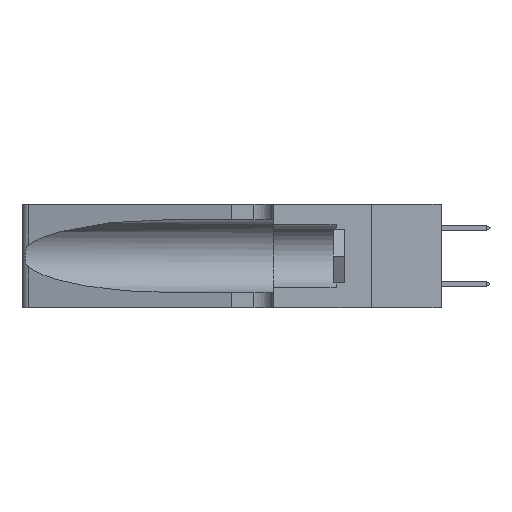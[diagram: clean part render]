
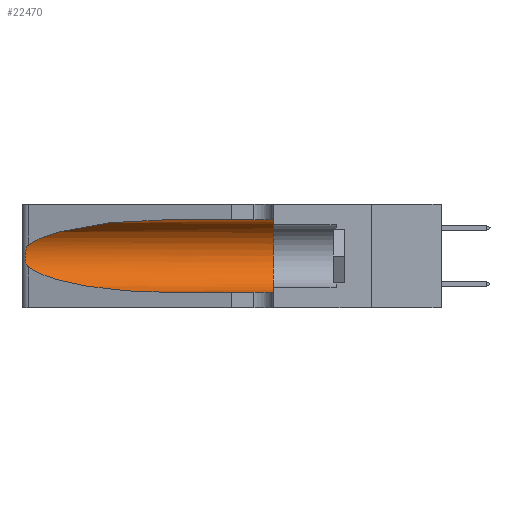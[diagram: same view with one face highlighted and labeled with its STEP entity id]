
A CAD part, left-side view. The second image highlights one B-rep face of the part: STEP entity #22470.
In plain terms, the highlighted cylindrical face has radius 3.308 mm (diameter 6.617 mm), a partial arc.
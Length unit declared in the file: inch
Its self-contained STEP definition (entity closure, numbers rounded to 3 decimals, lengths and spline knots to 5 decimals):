
#306 = EDGE_CURVE ( 'NONE', #28174, #3345, #5895, .T. ) ;
#857 = CARTESIAN_POINT ( 'NONE',  ( 0.1305, 0.72297, 0.31525 ) ) ;
#1840 = VERTEX_POINT ( 'NONE', #23225 ) ;
#2277 = CARTESIAN_POINT ( 'NONE',  ( 0.18966, 0.96281, 0.31525 ) ) ;
#3060 = CARTESIAN_POINT ( 'NONE',  ( 0.18966, 0.96281, 0.05475 ) ) ;
#3345 = VERTEX_POINT ( 'NONE', #25673 ) ;
#3553 = B_SPLINE_CURVE_WITH_KNOTS ( 'NONE', 3,
 ( #9175, #27335, #27452, #32509, #19311, #3940, #24472, #3828, #27086, #4163, #21787, #6830, #11520, #24708 ),
 .UNSPECIFIED., .F., .F.,
 ( 4, 2, 2, 2, 2, 2, 4 ),
 ( 0., 0.00027, 0.00053, 0.00107, 0.0016, 0.00187, 0.00214 ),
 .UNSPECIFIED. ) ;
#3712 = EDGE_CURVE ( 'NONE', #15146, #7098, #31193, .T. ) ;
#3828 = CARTESIAN_POINT ( 'NONE',  ( 0.26075, 1.23896, 0.178 ) ) ;
#3871 = DIRECTION ( 'NONE',  ( 0., -1., 0. ) ) ;
#3940 = CARTESIAN_POINT ( 'NONE',  ( 0.26018, 1.23835, 0.19895 ) ) ;
#4018 = EDGE_CURVE ( 'NONE', #1840, #28174, #20892, .T. ) ;
#4163 = CARTESIAN_POINT ( 'NONE',  ( 0.25856, 1.23593, 0.16098 ) ) ;
#4783 = VECTOR ( 'NONE', #17053, 39.37008 ) ;
#4831 = DIRECTION ( 'NONE',  ( 0., 0., 1. ) ) ;
#5895 = LINE ( 'NONE', #30026, #27263 ) ;
#6830 = CARTESIAN_POINT ( 'NONE',  ( 0.25639, 1.23186, 0.15144 ) ) ;
#6967 = ORIENTED_EDGE ( 'NONE', *, *, #7534, .F. ) ;
#7098 = VERTEX_POINT ( 'NONE', #7559 ) ;
#7534 = EDGE_CURVE ( 'NONE', #15146, #12720, #18056, .T. ) ;
#7559 = CARTESIAN_POINT ( 'NONE',  ( 0.25487, 1.22718, 0.22369 ) ) ;
#8106 = ORIENTED_EDGE ( 'NONE', *, *, #31319, .T. ) ;
#9175 = CARTESIAN_POINT ( 'NONE',  ( 0.25487, 1.22718, 0.22369 ) ) ;
#9202 = CARTESIAN_POINT ( 'NONE',  ( 0.1305, 0.72297, 0.05475 ) ) ;
#9577 = CARTESIAN_POINT ( 'NONE',  ( 0.1305, 0.72297, 0.31525 ) ) ;
#9977 = CYLINDRICAL_SURFACE ( 'NONE', #10581, 0.13025 ) ;
#10581 = AXIS2_PLACEMENT_3D ( 'NONE', #27297, #11972, #20083 ) ;
#11520 = CARTESIAN_POINT ( 'NONE',  ( 0.25555, 1.22993, 0.14849 ) ) ;
#11631 = CARTESIAN_POINT ( 'NONE',  ( 0.25487, 1.22718, 0.14631 ) ) ;
#11972 = DIRECTION ( 'NONE',  ( 0., -1., 0. ) ) ;
#12385 = CARTESIAN_POINT ( 'NONE',  ( 0.25487, 1.22718, 0.22369 ) ) ;
#12720 = VERTEX_POINT ( 'NONE', #24852 ) ;
#13055 = ORIENTED_EDGE ( 'NONE', *, *, #20165, .F. ) ;
#14045 = CIRCLE ( 'NONE', #21996, 0.13025 ) ;
#15146 = VERTEX_POINT ( 'NONE', #857 ) ;
#15517 = CARTESIAN_POINT ( 'NONE',  ( 0.1305, 0.72297, 0.05475 ) ) ;
#17053 = DIRECTION ( 'NONE',  ( 0., -1., 0. ) ) ;
#17413 = CARTESIAN_POINT ( 'NONE',  ( 0.1305, 0.35, 0.185 ) ) ;
#18056 = LINE ( 'NONE', #27309, #4783 ) ;
#19311 = CARTESIAN_POINT ( 'NONE',  ( 0.25854, 1.2359, 0.20912 ) ) ;
#20083 = DIRECTION ( 'NONE',  ( 0., 0., -1. ) ) ;
#20165 = EDGE_CURVE ( 'NONE', #12720, #3345, #14045, .T. ) ;
#20892 =( BOUNDED_CURVE ( )  B_SPLINE_CURVE ( 3, ( #11631, #28710, #3060, #9202 ),
 .UNSPECIFIED., .F., .F. ) 
 B_SPLINE_CURVE_WITH_KNOTS ( ( 4, 4 ),
 ( 3.44316, 4.71239 ),
 .UNSPECIFIED. ) 
 CURVE ( )  GEOMETRIC_REPRESENTATION_ITEM ( )  RATIONAL_B_SPLINE_CURVE ( ( 1., 0.87, 0.87, 1. ) ) 
 REPRESENTATION_ITEM ( '' )  );
#21787 = CARTESIAN_POINT ( 'NONE',  ( 0.25789, 1.23486, 0.15765 ) ) ;
#21996 = AXIS2_PLACEMENT_3D ( 'NONE', #17413, #25295, #4831 ) ;
#22084 = ORIENTED_EDGE ( 'NONE', *, *, #3712, .T. ) ;
#22470 = ADVANCED_FACE ( 'NONE', ( #31660 ), #9977, .F. ) ;
#23225 = CARTESIAN_POINT ( 'NONE',  ( 0.25487, 1.22718, 0.14631 ) ) ;
#23958 = EDGE_LOOP ( 'NONE', ( #22084, #8106, #33043, #31104, #13055, #6967 ) ) ;
#24472 = CARTESIAN_POINT ( 'NONE',  ( 0.26075, 1.23896, 0.19203 ) ) ;
#24708 = CARTESIAN_POINT ( 'NONE',  ( 0.25487, 1.22718, 0.14631 ) ) ;
#24852 = CARTESIAN_POINT ( 'NONE',  ( 0.1305, 0.35, 0.31525 ) ) ;
#25295 = DIRECTION ( 'NONE',  ( 0., 1., 0. ) ) ;
#25673 = CARTESIAN_POINT ( 'NONE',  ( 0.1305, 0.35, 0.05475 ) ) ;
#27086 = CARTESIAN_POINT ( 'NONE',  ( 0.26017, 1.23833, 0.17102 ) ) ;
#27263 = VECTOR ( 'NONE', #3871, 39.37008 ) ;
#27297 = CARTESIAN_POINT ( 'NONE',  ( 0.1305, 1.61858, 0.185 ) ) ;
#27309 = CARTESIAN_POINT ( 'NONE',  ( 0.1305, 1.61858, 0.31525 ) ) ;
#27335 = CARTESIAN_POINT ( 'NONE',  ( 0.25555, 1.22994, 0.2215 ) ) ;
#27452 = CARTESIAN_POINT ( 'NONE',  ( 0.25639, 1.23184, 0.21858 ) ) ;
#28174 = VERTEX_POINT ( 'NONE', #15517 ) ;
#28710 = CARTESIAN_POINT ( 'NONE',  ( 0.2373, 1.15595, 0.08982 ) ) ;
#30026 = CARTESIAN_POINT ( 'NONE',  ( 0.1305, 1.61858, 0.05475 ) ) ;
#31104 = ORIENTED_EDGE ( 'NONE', *, *, #306, .T. ) ;
#31193 =( BOUNDED_CURVE ( )  B_SPLINE_CURVE ( 3, ( #9577, #2277, #32891, #12385 ),
 .UNSPECIFIED., .F., .F. ) 
 B_SPLINE_CURVE_WITH_KNOTS ( ( 4, 4 ),
 ( 1.5708, 2.84003 ),
 .UNSPECIFIED. ) 
 CURVE ( )  GEOMETRIC_REPRESENTATION_ITEM ( )  RATIONAL_B_SPLINE_CURVE ( ( 1., 0.87, 0.87, 1. ) ) 
 REPRESENTATION_ITEM ( '' )  );
#31319 = EDGE_CURVE ( 'NONE', #7098, #1840, #3553, .T. ) ;
#31660 = FACE_OUTER_BOUND ( 'NONE', #23958, .T. ) ;
#32509 = CARTESIAN_POINT ( 'NONE',  ( 0.25787, 1.23484, 0.2124 ) ) ;
#32891 = CARTESIAN_POINT ( 'NONE',  ( 0.2373, 1.15595, 0.28018 ) ) ;
#33043 = ORIENTED_EDGE ( 'NONE', *, *, #4018, .T. ) ;
